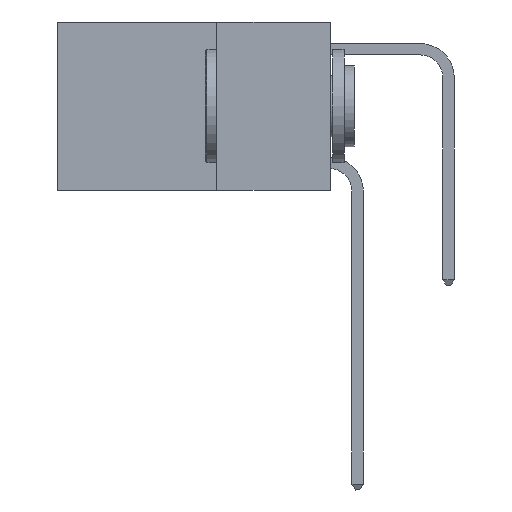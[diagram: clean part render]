
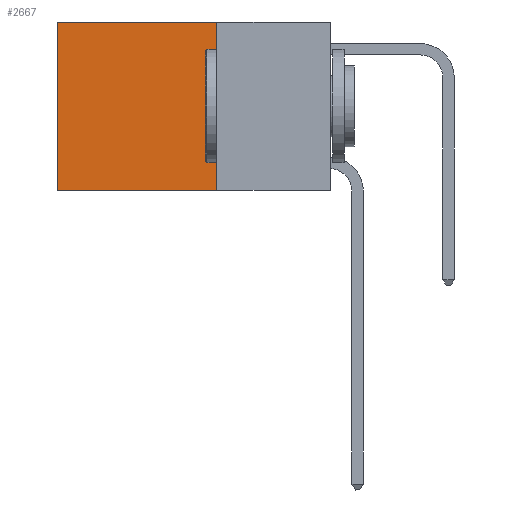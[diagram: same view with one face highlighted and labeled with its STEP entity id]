
A CAD part, left-side view. The second image highlights one B-rep face of the part: STEP entity #2667.
In plain terms, the highlighted planar face has unit normal (-1, 0, 0).
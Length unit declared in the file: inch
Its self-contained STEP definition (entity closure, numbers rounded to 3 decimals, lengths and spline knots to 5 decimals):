
#176 = CARTESIAN_POINT ( 'NONE',  ( 0.2625, 0.25, -0.37 ) ) ;
#883 = DIRECTION ( 'NONE',  ( 1., 0., 0. ) ) ;
#921 = CARTESIAN_POINT ( 'NONE',  ( 0.2625, 0.25, 0. ) ) ;
#1311 = VECTOR ( 'NONE', #10366, 39.37008 ) ;
#2326 = VECTOR ( 'NONE', #8797, 39.37008 ) ;
#2528 = CARTESIAN_POINT ( 'NONE',  ( 0.2625, 0.25, 0. ) ) ;
#2608 = ORIENTED_EDGE ( 'NONE', *, *, #9563, .T. ) ;
#2667 = ADVANCED_FACE ( 'NONE', ( #4041 ), #7998, .F. ) ;
#3051 = CARTESIAN_POINT ( 'NONE',  ( 0.2625, 0.6, -0.37 ) ) ;
#3190 = CARTESIAN_POINT ( 'NONE',  ( 0.2625, 0.25, -0.37 ) ) ;
#4041 = FACE_OUTER_BOUND ( 'NONE', #6808, .T. ) ;
#4603 = LINE ( 'NONE', #5244, #2326 ) ;
#4630 = DIRECTION ( 'NONE',  ( 0., 0., -1. ) ) ;
#5244 = CARTESIAN_POINT ( 'NONE',  ( 0.2625, 0.25, 0. ) ) ;
#6287 = CARTESIAN_POINT ( 'NONE',  ( 0.2625, 0.6, 0. ) ) ;
#6808 = EDGE_LOOP ( 'NONE', ( #13610, #9058, #15275, #2608 ) ) ;
#7065 = VERTEX_POINT ( 'NONE', #2528 ) ;
#7457 = DIRECTION ( 'NONE',  ( 0., 0., -1. ) ) ;
#7821 = LINE ( 'NONE', #176, #13402 ) ;
#7990 = VERTEX_POINT ( 'NONE', #3051 ) ;
#7998 = PLANE ( 'NONE',  #15129 ) ;
#8797 = DIRECTION ( 'NONE',  ( 0., 1., 0. ) ) ;
#9058 = ORIENTED_EDGE ( 'NONE', *, *, #14499, .F. ) ;
#9563 = EDGE_CURVE ( 'NONE', #7065, #11193, #4603, .T. ) ;
#10366 = DIRECTION ( 'NONE',  ( 0., 0., -1. ) ) ;
#11113 = VECTOR ( 'NONE', #7457, 39.37008 ) ;
#11193 = VERTEX_POINT ( 'NONE', #12864 ) ;
#11576 = CARTESIAN_POINT ( 'NONE',  ( 0.2625, 0.25, 0. ) ) ;
#12426 = VERTEX_POINT ( 'NONE', #3190 ) ;
#12638 = LINE ( 'NONE', #6287, #11113 ) ;
#12864 = CARTESIAN_POINT ( 'NONE',  ( 0.2625, 0.6, 0. ) ) ;
#13402 = VECTOR ( 'NONE', #14241, 39.37008 ) ;
#13610 = ORIENTED_EDGE ( 'NONE', *, *, #14720, .T. ) ;
#13915 = EDGE_CURVE ( 'NONE', #7065, #12426, #15081, .T. ) ;
#14241 = DIRECTION ( 'NONE',  ( 0., 1., 0. ) ) ;
#14499 = EDGE_CURVE ( 'NONE', #12426, #7990, #7821, .T. ) ;
#14720 = EDGE_CURVE ( 'NONE', #11193, #7990, #12638, .T. ) ;
#15081 = LINE ( 'NONE', #921, #1311 ) ;
#15129 = AXIS2_PLACEMENT_3D ( 'NONE', #11576, #883, #4630 ) ;
#15275 = ORIENTED_EDGE ( 'NONE', *, *, #13915, .F. ) ;
